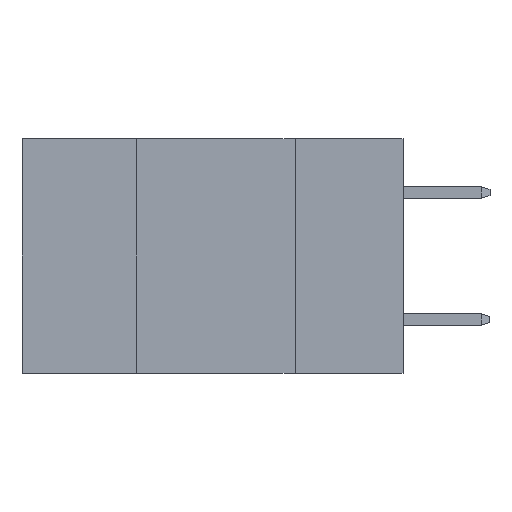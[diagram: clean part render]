
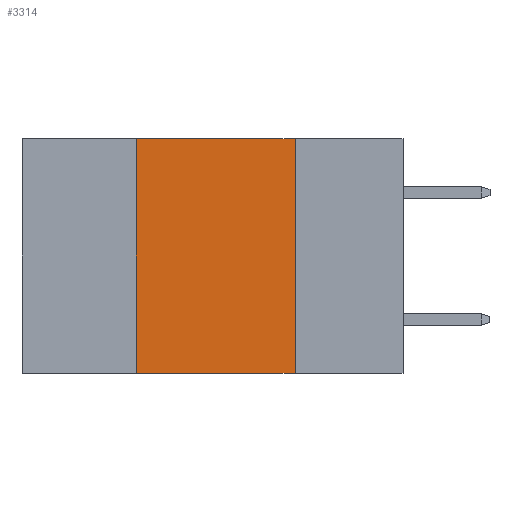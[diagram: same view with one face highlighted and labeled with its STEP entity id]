
A CAD part, left-side view. The second image highlights one B-rep face of the part: STEP entity #3314.
In plain terms, the highlighted planar face has unit normal (-1, 0, 0).
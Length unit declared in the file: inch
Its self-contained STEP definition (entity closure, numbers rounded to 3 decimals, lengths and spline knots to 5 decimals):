
#204 = DIRECTION ( 'NONE',  ( 0., -1., 0. ) ) ;
#263 = LINE ( 'NONE', #7433, #1156 ) ;
#484 = DIRECTION ( 'NONE',  ( 0., 0., 1. ) ) ;
#708 = DIRECTION ( 'NONE',  ( 0., -1., 0. ) ) ;
#773 = ORIENTED_EDGE ( 'NONE', *, *, #7064, .T. ) ;
#1156 = VECTOR ( 'NONE', #204, 39.37008 ) ;
#1256 = PLANE ( 'NONE',  #3343 ) ;
#1271 = CARTESIAN_POINT ( 'NONE',  ( 0., 0.17, 0. ) ) ;
#1464 = CARTESIAN_POINT ( 'NONE',  ( 0., 0.42, -0.37 ) ) ;
#1894 = CARTESIAN_POINT ( 'NONE',  ( 0., 0.6, 0. ) ) ;
#2053 = CARTESIAN_POINT ( 'NONE',  ( 0., 0.42, 0. ) ) ;
#2652 = VECTOR ( 'NONE', #484, 39.37008 ) ;
#2756 = CARTESIAN_POINT ( 'NONE',  ( 0., 0.42, 0. ) ) ;
#3248 = ORIENTED_EDGE ( 'NONE', *, *, #5472, .F. ) ;
#3251 = EDGE_CURVE ( 'NONE', #8219, #3282, #9288, .T. ) ;
#3282 = VERTEX_POINT ( 'NONE', #2053 ) ;
#3314 = ADVANCED_FACE ( 'NONE', ( #5909 ), #1256, .F. ) ;
#3343 = AXIS2_PLACEMENT_3D ( 'NONE', #1894, #8362, #6526 ) ;
#3580 = EDGE_CURVE ( 'NONE', #3282, #9481, #263, .T. ) ;
#4503 = DIRECTION ( 'NONE',  ( 0., 0., -1. ) ) ;
#5472 = EDGE_CURVE ( 'NONE', #9481, #5850, #6474, .T. ) ;
#5757 = CARTESIAN_POINT ( 'NONE',  ( 0., 0.17, -0.37 ) ) ;
#5850 = VERTEX_POINT ( 'NONE', #5757 ) ;
#5909 = FACE_OUTER_BOUND ( 'NONE', #9562, .T. ) ;
#6321 = ORIENTED_EDGE ( 'NONE', *, *, #3580, .F. ) ;
#6474 = LINE ( 'NONE', #9259, #8247 ) ;
#6526 = DIRECTION ( 'NONE',  ( 0., 0., -1. ) ) ;
#7064 = EDGE_CURVE ( 'NONE', #8219, #5850, #8755, .T. ) ;
#7336 = ORIENTED_EDGE ( 'NONE', *, *, #3251, .F. ) ;
#7433 = CARTESIAN_POINT ( 'NONE',  ( 0., 0.6, 0. ) ) ;
#7953 = CARTESIAN_POINT ( 'NONE',  ( 0., 0.6, -0.37 ) ) ;
#8219 = VERTEX_POINT ( 'NONE', #1464 ) ;
#8247 = VECTOR ( 'NONE', #4503, 39.37008 ) ;
#8362 = DIRECTION ( 'NONE',  ( 1., 0., 0. ) ) ;
#8755 = LINE ( 'NONE', #7953, #10137 ) ;
#9259 = CARTESIAN_POINT ( 'NONE',  ( 0., 0.17, 0. ) ) ;
#9288 = LINE ( 'NONE', #2756, #2652 ) ;
#9481 = VERTEX_POINT ( 'NONE', #1271 ) ;
#9562 = EDGE_LOOP ( 'NONE', ( #3248, #6321, #7336, #773 ) ) ;
#10137 = VECTOR ( 'NONE', #708, 39.37008 ) ;
